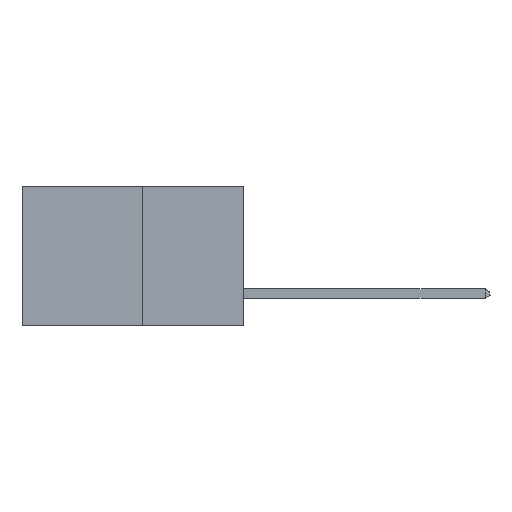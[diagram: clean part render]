
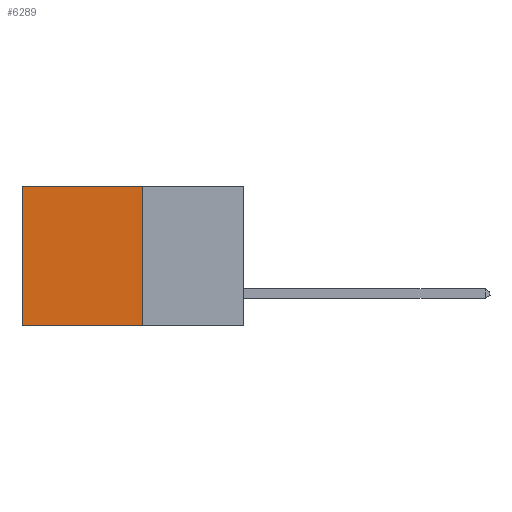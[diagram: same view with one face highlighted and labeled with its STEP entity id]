
A CAD part, left-side view. The second image highlights one B-rep face of the part: STEP entity #6289.
In plain terms, the highlighted planar face has unit normal (-1, 0, 0).
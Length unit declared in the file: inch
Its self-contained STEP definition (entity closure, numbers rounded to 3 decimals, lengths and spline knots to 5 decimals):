
#288 = LINE ( 'NONE', #7666, #4238 ) ;
#455 = EDGE_CURVE ( 'NONE', #4419, #4675, #5772, .T. ) ;
#619 = ORIENTED_EDGE ( 'NONE', *, *, #455, .F. ) ;
#1477 = CARTESIAN_POINT ( 'NONE',  ( 0.277, 0.59, 0. ) ) ;
#1631 = PLANE ( 'NONE',  #3500 ) ;
#2082 = LINE ( 'NONE', #3814, #4570 ) ;
#2437 = DIRECTION ( 'NONE',  ( 0., 0., -1. ) ) ;
#2649 = VECTOR ( 'NONE', #8733, 39.37008 ) ;
#2763 = DIRECTION ( 'NONE',  ( 0., 1., 0. ) ) ;
#2839 = EDGE_CURVE ( 'NONE', #4675, #9954, #2082, .T. ) ;
#3084 = VERTEX_POINT ( 'NONE', #1477 ) ;
#3395 = CARTESIAN_POINT ( 'NONE',  ( 0.277, 0.59, -0.37 ) ) ;
#3500 = AXIS2_PLACEMENT_3D ( 'NONE', #5769, #7383, #2437 ) ;
#3802 = DIRECTION ( 'NONE',  ( 0., 1., 0. ) ) ;
#3806 = EDGE_LOOP ( 'NONE', ( #10588, #5697, #619, #7593 ) ) ;
#3814 = CARTESIAN_POINT ( 'NONE',  ( 0.277, 0.27, -0.37 ) ) ;
#3821 = CARTESIAN_POINT ( 'NONE',  ( 0.277, 0.59, -0.37 ) ) ;
#4143 = CARTESIAN_POINT ( 'NONE',  ( 0.277, 0.27, -0.37 ) ) ;
#4238 = VECTOR ( 'NONE', #2763, 39.37008 ) ;
#4419 = VERTEX_POINT ( 'NONE', #6022 ) ;
#4570 = VECTOR ( 'NONE', #3802, 39.37008 ) ;
#4675 = VERTEX_POINT ( 'NONE', #4143 ) ;
#4926 = FACE_OUTER_BOUND ( 'NONE', #3806, .T. ) ;
#5697 = ORIENTED_EDGE ( 'NONE', *, *, #2839, .F. ) ;
#5769 = CARTESIAN_POINT ( 'NONE',  ( 0.277, 0.27, -0.37 ) ) ;
#5772 = LINE ( 'NONE', #8336, #9569 ) ;
#6022 = CARTESIAN_POINT ( 'NONE',  ( 0.277, 0.27, 0. ) ) ;
#6289 = ADVANCED_FACE ( 'NONE', ( #4926 ), #1631, .F. ) ;
#6542 = EDGE_CURVE ( 'NONE', #4419, #3084, #288, .T. ) ;
#6713 = EDGE_CURVE ( 'NONE', #3084, #9954, #7047, .T. ) ;
#7047 = LINE ( 'NONE', #3821, #2649 ) ;
#7383 = DIRECTION ( 'NONE',  ( 1., 0., 0. ) ) ;
#7593 = ORIENTED_EDGE ( 'NONE', *, *, #6542, .T. ) ;
#7666 = CARTESIAN_POINT ( 'NONE',  ( 0.277, 0.27, 0. ) ) ;
#8336 = CARTESIAN_POINT ( 'NONE',  ( 0.277, 0.27, -0.37 ) ) ;
#8733 = DIRECTION ( 'NONE',  ( 0., 0., -1. ) ) ;
#9569 = VECTOR ( 'NONE', #10567, 39.37008 ) ;
#9954 = VERTEX_POINT ( 'NONE', #3395 ) ;
#10567 = DIRECTION ( 'NONE',  ( 0., 0., -1. ) ) ;
#10588 = ORIENTED_EDGE ( 'NONE', *, *, #6713, .T. ) ;
